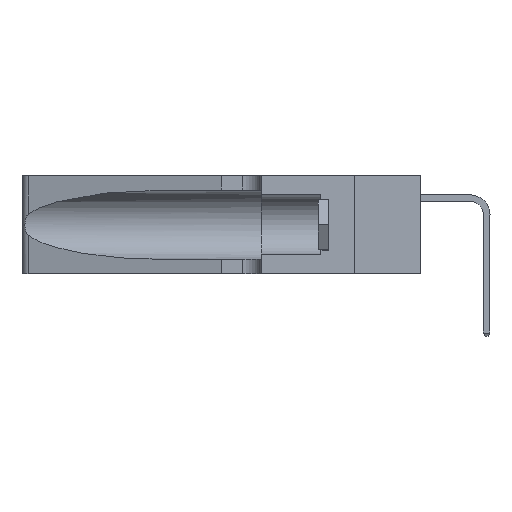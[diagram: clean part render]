
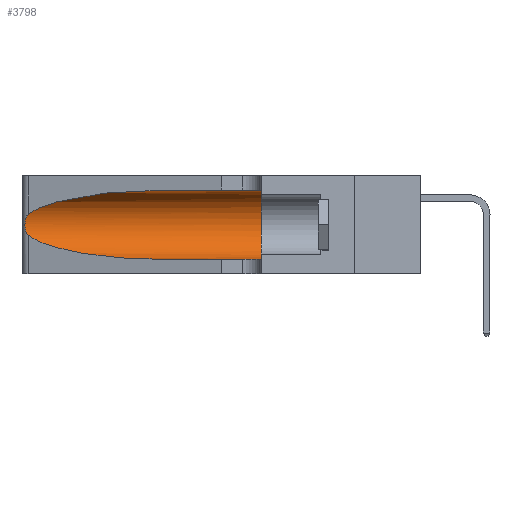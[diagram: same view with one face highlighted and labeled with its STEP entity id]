
A CAD part, left-side view. The second image highlights one B-rep face of the part: STEP entity #3798.
In plain terms, the highlighted cylindrical face has radius 3.308 mm (diameter 6.617 mm), a partial arc.
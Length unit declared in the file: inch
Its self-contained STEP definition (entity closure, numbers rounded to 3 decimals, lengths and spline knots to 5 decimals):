
#186 = DIRECTION ( 'NONE',  ( 0., 0., -1. ) ) ;
#247 = EDGE_CURVE ( 'NONE', #24611, #11117, #24578, .T. ) ;
#567 = CARTESIAN_POINT ( 'NONE',  ( 0.26075, 1.23896, 0.19203 ) ) ;
#859 =( BOUNDED_CURVE ( )  B_SPLINE_CURVE ( 3, ( #21257, #3344, #27948, #14600 ),
 .UNSPECIFIED., .F., .F. ) 
 B_SPLINE_CURVE_WITH_KNOTS ( ( 4, 4 ),
 ( 1.5708, 2.84003 ),
 .UNSPECIFIED. ) 
 CURVE ( )  GEOMETRIC_REPRESENTATION_ITEM ( )  RATIONAL_B_SPLINE_CURVE ( ( 1., 0.87, 0.87, 1. ) ) 
 REPRESENTATION_ITEM ( '' )  );
#1302 = CARTESIAN_POINT ( 'NONE',  ( 0.1305, 0.72297, 0.05475 ) ) ;
#1865 = DIRECTION ( 'NONE',  ( 0., -1., 0. ) ) ;
#1962 = CARTESIAN_POINT ( 'NONE',  ( 0.25487, 1.22718, 0.22369 ) ) ;
#2349 = CARTESIAN_POINT ( 'NONE',  ( 0.1305, 0.35, 0.05475 ) ) ;
#3344 = CARTESIAN_POINT ( 'NONE',  ( 0.18966, 0.96281, 0.31525 ) ) ;
#3748 = CARTESIAN_POINT ( 'NONE',  ( 0.25555, 1.22994, 0.2215 ) ) ;
#3798 = ADVANCED_FACE ( 'NONE', ( #17092 ), #16375, .F. ) ;
#3841 = VERTEX_POINT ( 'NONE', #7051 ) ;
#3919 = DIRECTION ( 'NONE',  ( 0., 1., 0. ) ) ;
#4526 = ORIENTED_EDGE ( 'NONE', *, *, #6862, .T. ) ;
#6379 = AXIS2_PLACEMENT_3D ( 'NONE', #11361, #24733, #186 ) ;
#6862 = EDGE_CURVE ( 'NONE', #21376, #14433, #15298, .T. ) ;
#7051 = CARTESIAN_POINT ( 'NONE',  ( 0.1305, 0.35, 0.31525 ) ) ;
#7963 = CARTESIAN_POINT ( 'NONE',  ( 0.25487, 1.22718, 0.14631 ) ) ;
#8855 = CARTESIAN_POINT ( 'NONE',  ( 0.25854, 1.2359, 0.20912 ) ) ;
#8913 = CARTESIAN_POINT ( 'NONE',  ( 0.26018, 1.23835, 0.19895 ) ) ;
#9358 = VECTOR ( 'NONE', #1865, 39.37008 ) ;
#10078 = ORIENTED_EDGE ( 'NONE', *, *, #25977, .T. ) ;
#11117 = VERTEX_POINT ( 'NONE', #28424 ) ;
#11361 = CARTESIAN_POINT ( 'NONE',  ( 0.1305, 1.61858, 0.185 ) ) ;
#12052 = ORIENTED_EDGE ( 'NONE', *, *, #27737, .T. ) ;
#13793 = CARTESIAN_POINT ( 'NONE',  ( 0.25487, 1.22718, 0.14631 ) ) ;
#13917 = CARTESIAN_POINT ( 'NONE',  ( 0.26017, 1.23833, 0.17102 ) ) ;
#14433 = VERTEX_POINT ( 'NONE', #2349 ) ;
#14600 = CARTESIAN_POINT ( 'NONE',  ( 0.25487, 1.22718, 0.22369 ) ) ;
#14609 = CARTESIAN_POINT ( 'NONE',  ( 0.25555, 1.22993, 0.14849 ) ) ;
#14649 = CARTESIAN_POINT ( 'NONE',  ( 0.25856, 1.23593, 0.16098 ) ) ;
#14673 = CARTESIAN_POINT ( 'NONE',  ( 0.25639, 1.23186, 0.15144 ) ) ;
#14695 = CARTESIAN_POINT ( 'NONE',  ( 0.18966, 0.96281, 0.05475 ) ) ;
#14990 = CARTESIAN_POINT ( 'NONE',  ( 0.1305, 1.61858, 0.31525 ) ) ;
#15169 =( BOUNDED_CURVE ( )  B_SPLINE_CURVE ( 3, ( #7963, #25839, #14695, #1302 ),
 .UNSPECIFIED., .F., .F. ) 
 B_SPLINE_CURVE_WITH_KNOTS ( ( 4, 4 ),
 ( 3.44316, 4.71239 ),
 .UNSPECIFIED. ) 
 CURVE ( )  GEOMETRIC_REPRESENTATION_ITEM ( )  RATIONAL_B_SPLINE_CURVE ( ( 1., 0.87, 0.87, 1. ) ) 
 REPRESENTATION_ITEM ( '' )  );
#15298 = LINE ( 'NONE', #24141, #9358 ) ;
#15505 = VERTEX_POINT ( 'NONE', #26160 ) ;
#16375 = CYLINDRICAL_SURFACE ( 'NONE', #6379, 0.13025 ) ;
#17092 = FACE_OUTER_BOUND ( 'NONE', #17257, .T. ) ;
#17241 = DIRECTION ( 'NONE',  ( 0., -1., 0. ) ) ;
#17246 = CIRCLE ( 'NONE', #28009, 0.13025 ) ;
#17257 = EDGE_LOOP ( 'NONE', ( #12052, #19741, #10078, #4526, #21265, #23150 ) ) ;
#17315 = CARTESIAN_POINT ( 'NONE',  ( 0.1305, 0.35, 0.185 ) ) ;
#18149 = VECTOR ( 'NONE', #17241, 39.37008 ) ;
#18566 = CARTESIAN_POINT ( 'NONE',  ( 0.25787, 1.23484, 0.2124 ) ) ;
#18982 = CARTESIAN_POINT ( 'NONE',  ( 0.25487, 1.22718, 0.22369 ) ) ;
#19168 = EDGE_CURVE ( 'NONE', #3841, #14433, #17246, .T. ) ;
#19552 = DIRECTION ( 'NONE',  ( 0., 0., 1. ) ) ;
#19741 = ORIENTED_EDGE ( 'NONE', *, *, #247, .T. ) ;
#20358 = CARTESIAN_POINT ( 'NONE',  ( 0.25639, 1.23184, 0.21858 ) ) ;
#21257 = CARTESIAN_POINT ( 'NONE',  ( 0.1305, 0.72297, 0.31525 ) ) ;
#21265 = ORIENTED_EDGE ( 'NONE', *, *, #19168, .F. ) ;
#21354 = CARTESIAN_POINT ( 'NONE',  ( 0.1305, 0.72297, 0.05475 ) ) ;
#21376 = VERTEX_POINT ( 'NONE', #21354 ) ;
#21502 = EDGE_CURVE ( 'NONE', #15505, #3841, #24089, .T. ) ;
#23150 = ORIENTED_EDGE ( 'NONE', *, *, #21502, .F. ) ;
#24089 = LINE ( 'NONE', #14990, #18149 ) ;
#24141 = CARTESIAN_POINT ( 'NONE',  ( 0.1305, 1.61858, 0.05475 ) ) ;
#24578 = B_SPLINE_CURVE_WITH_KNOTS ( 'NONE', 3,
 ( #18982, #3748, #20358, #18566, #8855, #8913, #567, #25910, #13917, #14649, #25984, #14673, #14609, #13793 ),
 .UNSPECIFIED., .F., .F.,
 ( 4, 2, 2, 2, 2, 2, 4 ),
 ( 0., 0.00027, 0.00053, 0.00107, 0.0016, 0.00187, 0.00214 ),
 .UNSPECIFIED. ) ;
#24611 = VERTEX_POINT ( 'NONE', #1962 ) ;
#24733 = DIRECTION ( 'NONE',  ( 0., -1., 0. ) ) ;
#25839 = CARTESIAN_POINT ( 'NONE',  ( 0.2373, 1.15595, 0.08982 ) ) ;
#25910 = CARTESIAN_POINT ( 'NONE',  ( 0.26075, 1.23896, 0.178 ) ) ;
#25977 = EDGE_CURVE ( 'NONE', #11117, #21376, #15169, .T. ) ;
#25984 = CARTESIAN_POINT ( 'NONE',  ( 0.25789, 1.23486, 0.15765 ) ) ;
#26160 = CARTESIAN_POINT ( 'NONE',  ( 0.1305, 0.72297, 0.31525 ) ) ;
#27737 = EDGE_CURVE ( 'NONE', #15505, #24611, #859, .T. ) ;
#27948 = CARTESIAN_POINT ( 'NONE',  ( 0.2373, 1.15595, 0.28018 ) ) ;
#28009 = AXIS2_PLACEMENT_3D ( 'NONE', #17315, #3919, #19552 ) ;
#28424 = CARTESIAN_POINT ( 'NONE',  ( 0.25487, 1.22718, 0.14631 ) ) ;
